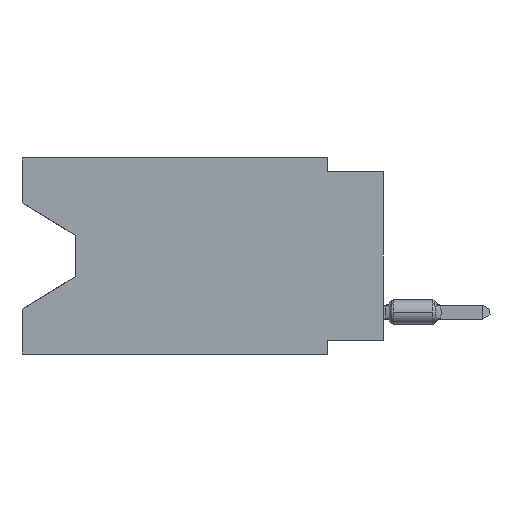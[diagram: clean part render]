
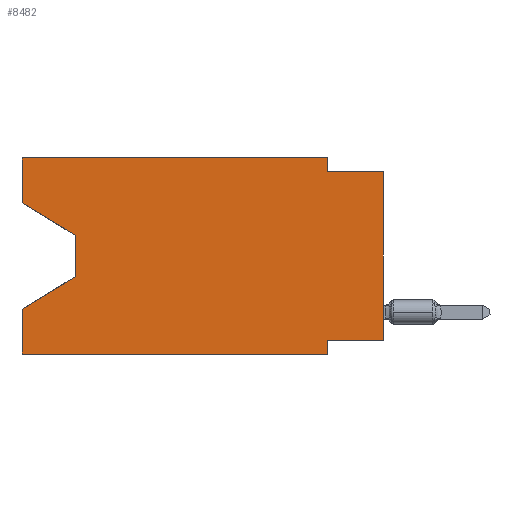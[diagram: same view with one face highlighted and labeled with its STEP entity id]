
A CAD part, left-side view. The second image highlights one B-rep face of the part: STEP entity #8482.
In plain terms, the highlighted planar face has unit normal (-1, 0, 0).
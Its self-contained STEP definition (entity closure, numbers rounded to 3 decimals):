
#85 = EDGE_CURVE ( 'NONE', #3479, #2789, #19275, .T. ) ;
#602 = CARTESIAN_POINT ( 'NONE',  ( 0., 16.383, 0. ) ) ;
#828 = LINE ( 'NONE', #5693, #2750 ) ;
#963 = CARTESIAN_POINT ( 'NONE',  ( 0., 16.383, 0. ) ) ;
#1072 = VERTEX_POINT ( 'NONE', #6163 ) ;
#1189 = DIRECTION ( 'NONE',  ( 0., -1., 0. ) ) ;
#1197 = ORIENTED_EDGE ( 'NONE', *, *, #7184, .T. ) ;
#1205 = DIRECTION ( 'NONE',  ( 0., -1., 0. ) ) ;
#1385 = CARTESIAN_POINT ( 'NONE',  ( 0., 13.97, -3.505 ) ) ;
#1437 = VERTEX_POINT ( 'NONE', #14189 ) ;
#1523 = EDGE_CURVE ( 'NONE', #20242, #5710, #20831, .T. ) ;
#2049 = VERTEX_POINT ( 'NONE', #16575 ) ;
#2148 = ORIENTED_EDGE ( 'NONE', *, *, #3690, .F. ) ;
#2553 = EDGE_CURVE ( 'NONE', #20242, #1072, #14911, .T. ) ;
#2750 = VECTOR ( 'NONE', #13634, 1000. ) ;
#2789 = VERTEX_POINT ( 'NONE', #20596 ) ;
#2983 = CARTESIAN_POINT ( 'NONE',  ( 0., 13.97, -3.505 ) ) ;
#3479 = VERTEX_POINT ( 'NONE', #10409 ) ;
#3690 = EDGE_CURVE ( 'NONE', #18028, #1072, #9130, .T. ) ;
#4183 = CARTESIAN_POINT ( 'NONE',  ( 0., 2.54, -8.255 ) ) ;
#4555 = EDGE_CURVE ( 'NONE', #14363, #18028, #16244, .T. ) ;
#4599 = VECTOR ( 'NONE', #1189, 1000. ) ;
#4861 = DIRECTION ( 'NONE',  ( 0., 1., 0. ) ) ;
#5118 = DIRECTION ( 'NONE',  ( 1., 0., 0. ) ) ;
#5246 = EDGE_CURVE ( 'NONE', #12691, #14363, #15667, .T. ) ;
#5693 = CARTESIAN_POINT ( 'NONE',  ( 0., 16.383, -2.038 ) ) ;
#5710 = VERTEX_POINT ( 'NONE', #4183 ) ;
#6061 = VERTEX_POINT ( 'NONE', #2983 ) ;
#6062 = LINE ( 'NONE', #15698, #17776 ) ;
#6163 = CARTESIAN_POINT ( 'NONE',  ( 0., 0., -0.635 ) ) ;
#6253 = CARTESIAN_POINT ( 'NONE',  ( 0., 13.97, -5.385 ) ) ;
#6486 = PLANE ( 'NONE',  #6740 ) ;
#6547 = DIRECTION ( 'NONE',  ( 0., 0., 1. ) ) ;
#6740 = AXIS2_PLACEMENT_3D ( 'NONE', #14747, #5118, #11249 ) ;
#6981 = DIRECTION ( 'NONE',  ( 0., 0., 1. ) ) ;
#7184 = EDGE_CURVE ( 'NONE', #3479, #12225, #6062, .T. ) ;
#7424 = DIRECTION ( 'NONE',  ( 0., -1., 0. ) ) ;
#7524 = DIRECTION ( 'NONE',  ( 0., 0., -1. ) ) ;
#7633 = CARTESIAN_POINT ( 'NONE',  ( 0., 2.54, -8.89 ) ) ;
#7732 = LINE ( 'NONE', #1385, #10181 ) ;
#8482 = ADVANCED_FACE ( 'NONE', ( #19288 ), #6486, .F. ) ;
#8745 = EDGE_CURVE ( 'NONE', #5710, #12225, #9221, .T. ) ;
#8983 = CARTESIAN_POINT ( 'NONE',  ( 0., 16.383, 0. ) ) ;
#9034 = VECTOR ( 'NONE', #6981, 1000. ) ;
#9040 = ORIENTED_EDGE ( 'NONE', *, *, #5246, .F. ) ;
#9130 = LINE ( 'NONE', #14098, #4599 ) ;
#9221 = LINE ( 'NONE', #7633, #11247 ) ;
#9471 = DIRECTION ( 'NONE',  ( 0., 0., -1. ) ) ;
#9522 = LINE ( 'NONE', #15971, #15255 ) ;
#9628 = ORIENTED_EDGE ( 'NONE', *, *, #85, .F. ) ;
#10181 = VECTOR ( 'NONE', #7524, 1000. ) ;
#10409 = CARTESIAN_POINT ( 'NONE',  ( 0., 16.383, -8.89 ) ) ;
#11033 = ORIENTED_EDGE ( 'NONE', *, *, #1523, .F. ) ;
#11096 = EDGE_LOOP ( 'NONE', ( #12124, #17791, #19968, #9628, #1197, #18497, #11033, #11962, #2148, #14410, #9040, #14797 ) ) ;
#11247 = VECTOR ( 'NONE', #17268, 1000. ) ;
#11249 = DIRECTION ( 'NONE',  ( 0., 0., -1. ) ) ;
#11319 = CARTESIAN_POINT ( 'NONE',  ( 0., 0., -8.255 ) ) ;
#11962 = ORIENTED_EDGE ( 'NONE', *, *, #2553, .T. ) ;
#12124 = ORIENTED_EDGE ( 'NONE', *, *, #15715, .T. ) ;
#12225 = VERTEX_POINT ( 'NONE', #18299 ) ;
#12691 = VERTEX_POINT ( 'NONE', #602 ) ;
#13634 = DIRECTION ( 'NONE',  ( 0., -0.855, -0.519 ) ) ;
#13827 = VECTOR ( 'NONE', #4861, 1000. ) ;
#14098 = CARTESIAN_POINT ( 'NONE',  ( 0., 0., -0.635 ) ) ;
#14189 = CARTESIAN_POINT ( 'NONE',  ( 0., 13.97, -5.385 ) ) ;
#14363 = VERTEX_POINT ( 'NONE', #17980 ) ;
#14410 = ORIENTED_EDGE ( 'NONE', *, *, #4555, .F. ) ;
#14747 = CARTESIAN_POINT ( 'NONE',  ( 0., 16.383, 0. ) ) ;
#14795 = VECTOR ( 'NONE', #18716, 1000. ) ;
#14797 = ORIENTED_EDGE ( 'NONE', *, *, #15561, .F. ) ;
#14911 = LINE ( 'NONE', #18195, #9034 ) ;
#15255 = VECTOR ( 'NONE', #6547, 1000. ) ;
#15561 = EDGE_CURVE ( 'NONE', #2049, #12691, #9522, .T. ) ;
#15667 = LINE ( 'NONE', #963, #19432 ) ;
#15698 = CARTESIAN_POINT ( 'NONE',  ( 0., 16.383, -8.89 ) ) ;
#15715 = EDGE_CURVE ( 'NONE', #2049, #6061, #828, .T. ) ;
#15827 = CARTESIAN_POINT ( 'NONE',  ( 0., 0., -8.255 ) ) ;
#15902 = LINE ( 'NONE', #6253, #20741 ) ;
#15971 = CARTESIAN_POINT ( 'NONE',  ( 0., 16.383, 0. ) ) ;
#16244 = LINE ( 'NONE', #18038, #17479 ) ;
#16575 = CARTESIAN_POINT ( 'NONE',  ( 0., 16.383, -2.038 ) ) ;
#16949 = CARTESIAN_POINT ( 'NONE',  ( 0., 2.54, -0.635 ) ) ;
#17013 = EDGE_CURVE ( 'NONE', #6061, #1437, #7732, .T. ) ;
#17268 = DIRECTION ( 'NONE',  ( 0., 0., -1. ) ) ;
#17479 = VECTOR ( 'NONE', #9471, 1000. ) ;
#17776 = VECTOR ( 'NONE', #1205, 1000. ) ;
#17791 = ORIENTED_EDGE ( 'NONE', *, *, #17013, .T. ) ;
#17980 = CARTESIAN_POINT ( 'NONE',  ( 0., 2.54, 0. ) ) ;
#18028 = VERTEX_POINT ( 'NONE', #16949 ) ;
#18038 = CARTESIAN_POINT ( 'NONE',  ( 0., 2.54, 0. ) ) ;
#18195 = CARTESIAN_POINT ( 'NONE',  ( 0., 0., 0. ) ) ;
#18299 = CARTESIAN_POINT ( 'NONE',  ( 0., 2.54, -8.89 ) ) ;
#18497 = ORIENTED_EDGE ( 'NONE', *, *, #8745, .F. ) ;
#18716 = DIRECTION ( 'NONE',  ( 0., 0., 1. ) ) ;
#18978 = EDGE_CURVE ( 'NONE', #1437, #2789, #15902, .T. ) ;
#19164 = DIRECTION ( 'NONE',  ( 0., 0.855, -0.519 ) ) ;
#19275 = LINE ( 'NONE', #8983, #14795 ) ;
#19288 = FACE_OUTER_BOUND ( 'NONE', #11096, .T. ) ;
#19432 = VECTOR ( 'NONE', #7424, 1000. ) ;
#19968 = ORIENTED_EDGE ( 'NONE', *, *, #18978, .T. ) ;
#20242 = VERTEX_POINT ( 'NONE', #15827 ) ;
#20596 = CARTESIAN_POINT ( 'NONE',  ( 0., 16.383, -6.852 ) ) ;
#20741 = VECTOR ( 'NONE', #19164, 1000. ) ;
#20831 = LINE ( 'NONE', #11319, #13827 ) ;
